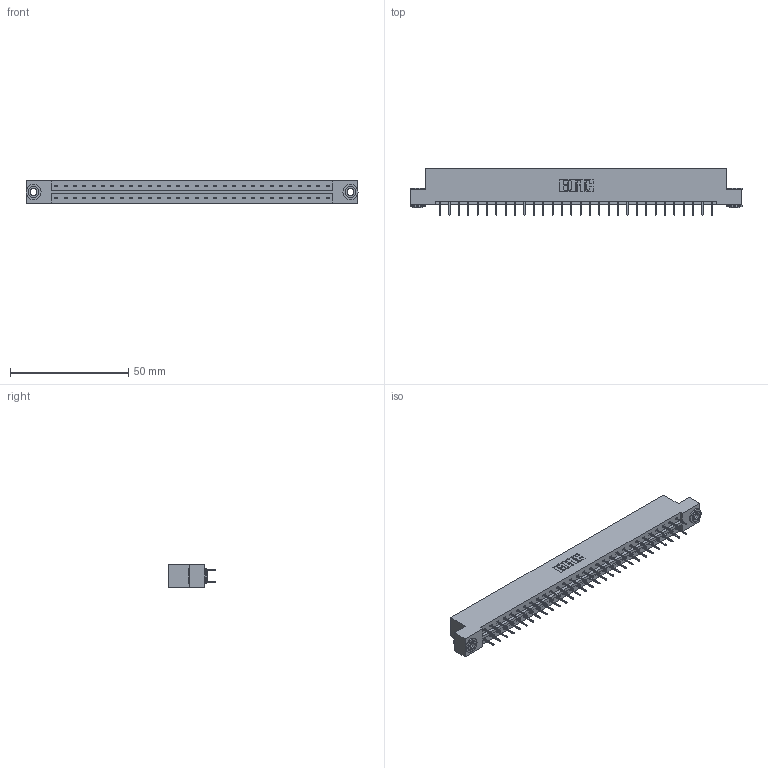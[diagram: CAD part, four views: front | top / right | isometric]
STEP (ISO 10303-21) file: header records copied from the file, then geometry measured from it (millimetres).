
FILE_DESCRIPTION (( 'STEP AP203' ), '1' );
FILE_NAME ('333-060-524-203.STEP', '2018-08-04T07:04:22', ( '' ), ( '' ), 'SwSTEP 2.0', 'SolidWorks 2016', '' );
FILE_SCHEMA (( 'CONFIG_CONTROL_DESIGN' ));
Length unit declared in the file: inch
Products named in the file (4): 333 Part_Flush - .156 Dia - TH; 345-292-001_345-293-124; 345-250-002_345-250-002-102; 333-060-524-203
Assembly tree (63 placements, depth 2):
  333-060-524-203
    333 Part_Flush - .156 Dia - TH
    345-292-001_345-293-124  x60
    345-250-002_345-250-002-102  x2
Bounding box: 140.41 x 19.69 x 9.4 mm (x, y, z)
Volume: 14151.6 mm3; surface area: 16550.1 mm2
Topology: 63 solids, 63 shells, 3512 faces, 9927 edges, 6374 vertices
Faces by surface type: plane 2600, cylinder 904, cone 8
Entity records: 21576 total; most frequent: CARTESIAN_POINT 3565, ORIENTED_EDGE 3494, DIRECTION 3101, EDGE_CURVE 1747, LINE 1599, VECTOR 1599, VERTEX_POINT 1158, AXIS2_PLACEMENT_3D 751
